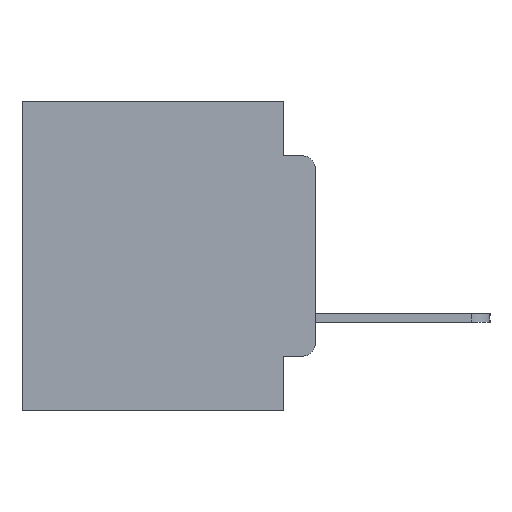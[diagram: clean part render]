
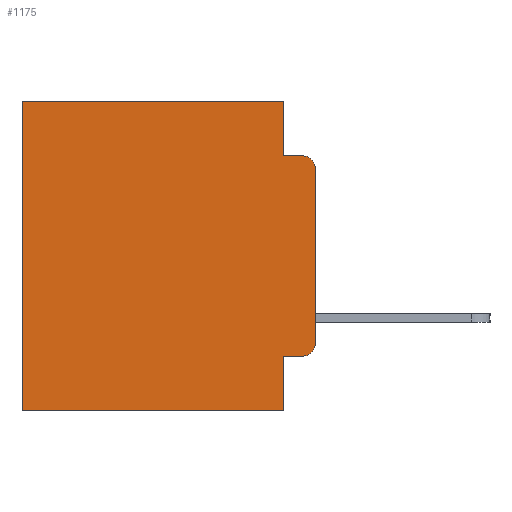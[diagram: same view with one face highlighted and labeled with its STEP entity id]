
A CAD part, left-side view. The second image highlights one B-rep face of the part: STEP entity #1175.
In plain terms, the highlighted planar face has unit normal (-1, 0, 0).
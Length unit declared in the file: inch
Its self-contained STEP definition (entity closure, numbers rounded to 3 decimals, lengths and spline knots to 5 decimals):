
#156 = CARTESIAN_POINT ( 'NONE',  ( 0.298, 0.051, 0. ) ) ;
#246 = ORIENTED_EDGE ( 'NONE', *, *, #7224, .F. ) ;
#760 = VERTEX_POINT ( 'NONE', #24083 ) ;
#956 = ORIENTED_EDGE ( 'NONE', *, *, #11869, .T. ) ;
#1078 = DIRECTION ( 'NONE',  ( 0., 1., 0. ) ) ;
#1159 = CARTESIAN_POINT ( 'NONE',  ( 0.298, 0., 0. ) ) ;
#1166 = EDGE_CURVE ( 'NONE', #4397, #760, #12235, .T. ) ;
#1175 = ADVANCED_FACE ( 'NONE', ( #4862 ), #18116, .F. ) ;
#1187 = ORIENTED_EDGE ( 'NONE', *, *, #6714, .F. ) ;
#1242 = LINE ( 'NONE', #1159, #21526 ) ;
#1719 = AXIS2_PLACEMENT_3D ( 'NONE', #18272, #18317, #18345 ) ;
#2103 = ORIENTED_EDGE ( 'NONE', *, *, #7459, .F. ) ;
#2614 = EDGE_CURVE ( 'NONE', #12288, #11401, #1242, .T. ) ;
#3736 = ORIENTED_EDGE ( 'NONE', *, *, #2614, .T. ) ;
#4397 = VERTEX_POINT ( 'NONE', #5638 ) ;
#4590 = VERTEX_POINT ( 'NONE', #19837 ) ;
#4670 = ORIENTED_EDGE ( 'NONE', *, *, #18215, .T. ) ;
#4862 = FACE_OUTER_BOUND ( 'NONE', #6933, .T. ) ;
#5420 = LINE ( 'NONE', #5666, #14864 ) ;
#5638 = CARTESIAN_POINT ( 'NONE',  ( 0.298, 0., -0.1085 ) ) ;
#5666 = CARTESIAN_POINT ( 'NONE',  ( 0.298, 0.051, 0. ) ) ;
#6090 = LINE ( 'NONE', #8234, #16661 ) ;
#6541 = ORIENTED_EDGE ( 'NONE', *, *, #16528, .T. ) ;
#6714 = EDGE_CURVE ( 'NONE', #4397, #11368, #6090, .T. ) ;
#6903 = CARTESIAN_POINT ( 'NONE',  ( 0.298, 0.02, -0.3915 ) ) ;
#6933 = EDGE_LOOP ( 'NONE', ( #1187, #9075, #8595, #7436, #3736, #6541, #2103, #246, #4670, #956 ) ) ;
#7224 = EDGE_CURVE ( 'NONE', #23918, #20920, #5420, .T. ) ;
#7436 = ORIENTED_EDGE ( 'NONE', *, *, #18978, .F. ) ;
#7459 = EDGE_CURVE ( 'NONE', #20920, #4590, #19239, .T. ) ;
#8059 = VECTOR ( 'NONE', #15873, 39.37008 ) ;
#8234 = CARTESIAN_POINT ( 'NONE',  ( 0.298, 0., 0. ) ) ;
#8595 = ORIENTED_EDGE ( 'NONE', *, *, #21423, .F. ) ;
#8641 = AXIS2_PLACEMENT_3D ( 'NONE', #18220, #18870, #19102 ) ;
#9000 = DIRECTION ( 'NONE',  ( 0., 0., -1. ) ) ;
#9075 = ORIENTED_EDGE ( 'NONE', *, *, #1166, .T. ) ;
#9215 = CARTESIAN_POINT ( 'NONE',  ( 0.298, 0., -0.3915 ) ) ;
#9834 = DIRECTION ( 'NONE',  ( 0., 0., -1. ) ) ;
#11364 = VERTEX_POINT ( 'NONE', #20646 ) ;
#11368 = VERTEX_POINT ( 'NONE', #9215 ) ;
#11401 = VERTEX_POINT ( 'NONE', #13316 ) ;
#11419 = DIRECTION ( 'NONE',  ( 0., -1., 0. ) ) ;
#11869 = EDGE_CURVE ( 'NONE', #15287, #11368, #17234, .T. ) ;
#12235 = CIRCLE ( 'NONE', #1719, 0.02 ) ;
#12288 = VERTEX_POINT ( 'NONE', #156 ) ;
#12302 = VECTOR ( 'NONE', #19001, 39.37008 ) ;
#13316 = CARTESIAN_POINT ( 'NONE',  ( 0.298, 0.473, 0. ) ) ;
#13704 = VECTOR ( 'NONE', #21955, 39.37008 ) ;
#13926 = CARTESIAN_POINT ( 'NONE',  ( 0.298, 0.051, -0.5 ) ) ;
#13953 = CARTESIAN_POINT ( 'NONE',  ( 0.298, 0.051, 0. ) ) ;
#14040 = LINE ( 'NONE', #13953, #8059 ) ;
#14864 = VECTOR ( 'NONE', #9834, 39.37008 ) ;
#14961 = VECTOR ( 'NONE', #23665, 39.37008 ) ;
#15287 = VERTEX_POINT ( 'NONE', #23115 ) ;
#15873 = DIRECTION ( 'NONE',  ( 0., 0., -1. ) ) ;
#16069 = LINE ( 'NONE', #20796, #20369 ) ;
#16528 = EDGE_CURVE ( 'NONE', #11401, #4590, #18489, .T. ) ;
#16661 = VECTOR ( 'NONE', #21607, 39.37008 ) ;
#17234 = CIRCLE ( 'NONE', #19984, 0.02 ) ;
#18116 = PLANE ( 'NONE',  #8641 ) ;
#18215 = EDGE_CURVE ( 'NONE', #23918, #15287, #19882, .T. ) ;
#18220 = CARTESIAN_POINT ( 'NONE',  ( 0.298, 0., 0. ) ) ;
#18272 = CARTESIAN_POINT ( 'NONE',  ( 0.298, 0.02, -0.1085 ) ) ;
#18317 = DIRECTION ( 'NONE',  ( -1., 0., 0. ) ) ;
#18345 = DIRECTION ( 'NONE',  ( 0., 0., -1. ) ) ;
#18489 = LINE ( 'NONE', #20772, #12302 ) ;
#18870 = DIRECTION ( 'NONE',  ( 1., 0., 0. ) ) ;
#18978 = EDGE_CURVE ( 'NONE', #12288, #11364, #14040, .T. ) ;
#19001 = DIRECTION ( 'NONE',  ( 0., 0., -1. ) ) ;
#19102 = DIRECTION ( 'NONE',  ( 0., 0., -1. ) ) ;
#19239 = LINE ( 'NONE', #20146, #13704 ) ;
#19837 = CARTESIAN_POINT ( 'NONE',  ( 0.298, 0.473, -0.5 ) ) ;
#19882 = LINE ( 'NONE', #21888, #14961 ) ;
#19984 = AXIS2_PLACEMENT_3D ( 'NONE', #6903, #20475, #9000 ) ;
#20146 = CARTESIAN_POINT ( 'NONE',  ( 0.298, 0., -0.5 ) ) ;
#20369 = VECTOR ( 'NONE', #11419, 39.37008 ) ;
#20475 = DIRECTION ( 'NONE',  ( -1., 0., 0. ) ) ;
#20646 = CARTESIAN_POINT ( 'NONE',  ( 0.298, 0.051, -0.0885 ) ) ;
#20772 = CARTESIAN_POINT ( 'NONE',  ( 0.298, 0.473, 0. ) ) ;
#20796 = CARTESIAN_POINT ( 'NONE',  ( 0.298, 0.051, -0.0885 ) ) ;
#20920 = VERTEX_POINT ( 'NONE', #13926 ) ;
#21423 = EDGE_CURVE ( 'NONE', #11364, #760, #16069, .T. ) ;
#21526 = VECTOR ( 'NONE', #1078, 39.37008 ) ;
#21607 = DIRECTION ( 'NONE',  ( 0., 0., -1. ) ) ;
#21888 = CARTESIAN_POINT ( 'NONE',  ( 0.298, 0.051, -0.4115 ) ) ;
#21955 = DIRECTION ( 'NONE',  ( 0., 1., 0. ) ) ;
#23115 = CARTESIAN_POINT ( 'NONE',  ( 0.298, 0.02, -0.4115 ) ) ;
#23140 = CARTESIAN_POINT ( 'NONE',  ( 0.298, 0.051, -0.4115 ) ) ;
#23665 = DIRECTION ( 'NONE',  ( 0., -1., 0. ) ) ;
#23918 = VERTEX_POINT ( 'NONE', #23140 ) ;
#24083 = CARTESIAN_POINT ( 'NONE',  ( 0.298, 0.02, -0.0885 ) ) ;
